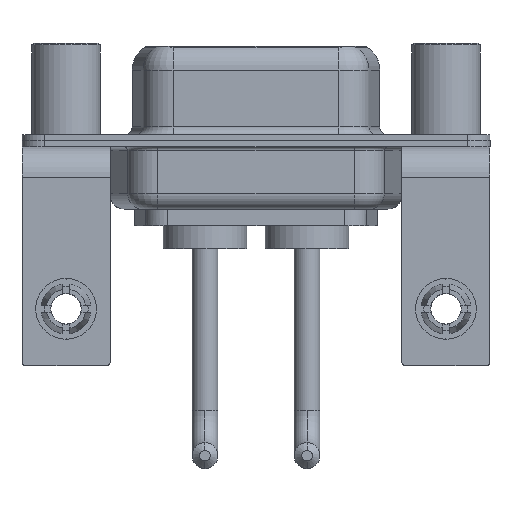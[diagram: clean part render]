
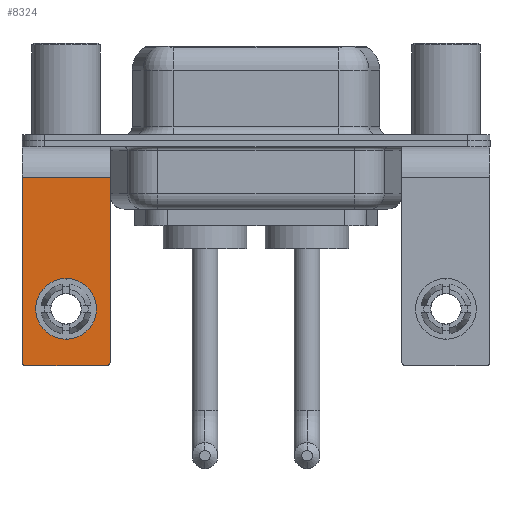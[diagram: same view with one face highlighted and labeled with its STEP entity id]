
A CAD part, front view. The second image highlights one B-rep face of the part: STEP entity #8324.
In plain terms, the highlighted planar face has unit normal (0, -1, 0).
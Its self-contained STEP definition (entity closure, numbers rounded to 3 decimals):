
#47 = DIRECTION ( 'NONE',  ( 0., 0., -1. ) ) ;
#170 = EDGE_CURVE ( 'NONE', #5880, #1158, #8578, .T. ) ;
#527 = CARTESIAN_POINT ( 'NONE',  ( 2.9, -6.25, -14.55 ) ) ;
#628 = CARTESIAN_POINT ( 'NONE',  ( 2.9, -6.25, -2.4 ) ) ;
#688 = EDGE_CURVE ( 'NONE', #10269, #6684, #8069, .T. ) ;
#957 = ORIENTED_EDGE ( 'NONE', *, *, #5173, .F. ) ;
#1024 = CARTESIAN_POINT ( 'NONE',  ( 0., -6.25, -13.07 ) ) ;
#1158 = VERTEX_POINT ( 'NONE', #1024 ) ;
#1207 = CARTESIAN_POINT ( 'NONE',  ( 2.65, -6.25, -14.8 ) ) ;
#1264 = DIRECTION ( 'NONE',  ( 0., -1., 0. ) ) ;
#1286 = AXIS2_PLACEMENT_3D ( 'NONE', #10815, #10887, #11046 ) ;
#1802 = CARTESIAN_POINT ( 'NONE',  ( 2.9, -6.25, -2.4 ) ) ;
#2009 = EDGE_CURVE ( 'NONE', #11478, #10269, #3334, .T. ) ;
#2553 = VECTOR ( 'NONE', #11841, 1000. ) ;
#2954 = DIRECTION ( 'NONE',  ( 0., 0., 1. ) ) ;
#3331 = EDGE_LOOP ( 'NONE', ( #3973, #14499 ) ) ;
#3334 = LINE ( 'NONE', #628, #11760 ) ;
#3411 = DIRECTION ( 'NONE',  ( -1., 0., 0. ) ) ;
#3723 = VERTEX_POINT ( 'NONE', #527 ) ;
#3973 = ORIENTED_EDGE ( 'NONE', *, *, #6423, .T. ) ;
#4018 = DIRECTION ( 'NONE',  ( 0., 1., 0. ) ) ;
#4526 = AXIS2_PLACEMENT_3D ( 'NONE', #14895, #14741, #9709 ) ;
#4617 = DIRECTION ( 'NONE',  ( 0., 1., 0. ) ) ;
#5173 = EDGE_CURVE ( 'NONE', #10167, #8190, #7044, .T. ) ;
#5187 = AXIS2_PLACEMENT_3D ( 'NONE', #13791, #1264, #7690 ) ;
#5243 = CARTESIAN_POINT ( 'NONE',  ( 0., -6.25, -11.07 ) ) ;
#5880 = VERTEX_POINT ( 'NONE', #13934 ) ;
#6423 = EDGE_CURVE ( 'NONE', #1158, #5880, #13978, .T. ) ;
#6684 = VERTEX_POINT ( 'NONE', #13818 ) ;
#7044 = LINE ( 'NONE', #12313, #8835 ) ;
#7294 = DIRECTION ( 'NONE',  ( -1., 0., 0. ) ) ;
#7398 = AXIS2_PLACEMENT_3D ( 'NONE', #5243, #4018, #2954 ) ;
#7690 = DIRECTION ( 'NONE',  ( 0., 0., 1. ) ) ;
#8031 = ORIENTED_EDGE ( 'NONE', *, *, #9685, .T. ) ;
#8069 = LINE ( 'NONE', #11860, #14395 ) ;
#8190 = VERTEX_POINT ( 'NONE', #14337 ) ;
#8324 = ADVANCED_FACE ( 'NONE', ( #9866, #13751 ), #8640, .F. ) ;
#8578 = CIRCLE ( 'NONE', #14891, 2. ) ;
#8628 = EDGE_CURVE ( 'NONE', #11478, #3723, #14398, .T. ) ;
#8640 = PLANE ( 'NONE',  #4526 ) ;
#8794 = ORIENTED_EDGE ( 'NONE', *, *, #2009, .T. ) ;
#8835 = VECTOR ( 'NONE', #7294, 1000. ) ;
#9414 = EDGE_CURVE ( 'NONE', #10167, #3723, #11253, .T. ) ;
#9685 = EDGE_CURVE ( 'NONE', #6684, #8190, #11002, .T. ) ;
#9709 = DIRECTION ( 'NONE',  ( 0., 0., 1. ) ) ;
#9866 = FACE_BOUND ( 'NONE', #3331, .T. ) ;
#10167 = VERTEX_POINT ( 'NONE', #1207 ) ;
#10269 = VERTEX_POINT ( 'NONE', #11331 ) ;
#10815 = CARTESIAN_POINT ( 'NONE',  ( -2.65, -6.25, -14.55 ) ) ;
#10887 = DIRECTION ( 'NONE',  ( 0., -1., 0. ) ) ;
#10901 = ORIENTED_EDGE ( 'NONE', *, *, #8628, .F. ) ;
#11002 = CIRCLE ( 'NONE', #1286, 0.25 ) ;
#11046 = DIRECTION ( 'NONE',  ( 0., 0., 1. ) ) ;
#11157 = ORIENTED_EDGE ( 'NONE', *, *, #688, .T. ) ;
#11253 = CIRCLE ( 'NONE', #5187, 0.25 ) ;
#11331 = CARTESIAN_POINT ( 'NONE',  ( -2.9, -6.25, -2.4 ) ) ;
#11478 = VERTEX_POINT ( 'NONE', #15342 ) ;
#11760 = VECTOR ( 'NONE', #3411, 1000. ) ;
#11841 = DIRECTION ( 'NONE',  ( 0., 0., -1. ) ) ;
#11860 = CARTESIAN_POINT ( 'NONE',  ( -2.9, -6.25, -2.4 ) ) ;
#12313 = CARTESIAN_POINT ( 'NONE',  ( 2.9, -6.25, -14.8 ) ) ;
#13133 = ORIENTED_EDGE ( 'NONE', *, *, #9414, .T. ) ;
#13751 = FACE_OUTER_BOUND ( 'NONE', #15542, .T. ) ;
#13791 = CARTESIAN_POINT ( 'NONE',  ( 2.65, -6.25, -14.55 ) ) ;
#13818 = CARTESIAN_POINT ( 'NONE',  ( -2.9, -6.25, -14.55 ) ) ;
#13934 = CARTESIAN_POINT ( 'NONE',  ( 0., -6.25, -9.07 ) ) ;
#13978 = CIRCLE ( 'NONE', #7398, 2. ) ;
#14337 = CARTESIAN_POINT ( 'NONE',  ( -2.65, -6.25, -14.8 ) ) ;
#14395 = VECTOR ( 'NONE', #47, 1000. ) ;
#14398 = LINE ( 'NONE', #1802, #2553 ) ;
#14499 = ORIENTED_EDGE ( 'NONE', *, *, #170, .T. ) ;
#14677 = DIRECTION ( 'NONE',  ( 0., 0., 1. ) ) ;
#14741 = DIRECTION ( 'NONE',  ( 0., 1., 0. ) ) ;
#14891 = AXIS2_PLACEMENT_3D ( 'NONE', #15938, #4617, #14677 ) ;
#14895 = CARTESIAN_POINT ( 'NONE',  ( 2.9, -6.25, -2.4 ) ) ;
#15342 = CARTESIAN_POINT ( 'NONE',  ( 2.9, -6.25, -2.4 ) ) ;
#15542 = EDGE_LOOP ( 'NONE', ( #11157, #8031, #957, #13133, #10901, #8794 ) ) ;
#15938 = CARTESIAN_POINT ( 'NONE',  ( 0., -6.25, -11.07 ) ) ;
